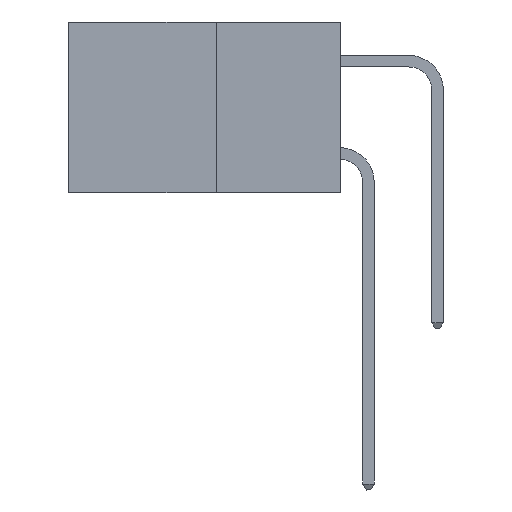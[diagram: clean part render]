
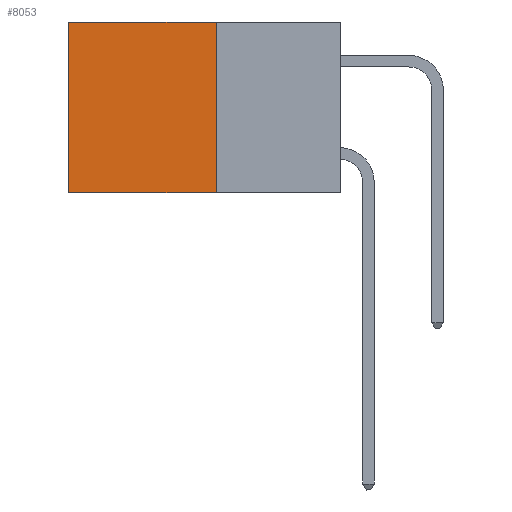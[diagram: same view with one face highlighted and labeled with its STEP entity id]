
A CAD part, left-side view. The second image highlights one B-rep face of the part: STEP entity #8053.
In plain terms, the highlighted planar face has unit normal (-1, 0, 0).
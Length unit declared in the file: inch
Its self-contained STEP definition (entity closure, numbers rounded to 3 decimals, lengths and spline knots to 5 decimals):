
#97 = CARTESIAN_POINT ( 'NONE',  ( 0.277, 0.59, 0. ) ) ;
#170 = EDGE_CURVE ( 'NONE', #8629, #263, #5665, .T. ) ;
#263 = VERTEX_POINT ( 'NONE', #1563 ) ;
#1008 = VECTOR ( 'NONE', #2138, 39.37008 ) ;
#1126 = ORIENTED_EDGE ( 'NONE', *, *, #170, .T. ) ;
#1205 = EDGE_LOOP ( 'NONE', ( #1126, #2444, #7667, #8447 ) ) ;
#1517 = VERTEX_POINT ( 'NONE', #9503 ) ;
#1563 = CARTESIAN_POINT ( 'NONE',  ( 0.277, 0.59, -0.37 ) ) ;
#2138 = DIRECTION ( 'NONE',  ( 0., 0., -1. ) ) ;
#2444 = ORIENTED_EDGE ( 'NONE', *, *, #2833, .F. ) ;
#2833 = EDGE_CURVE ( 'NONE', #4361, #263, #10148, .T. ) ;
#3329 = LINE ( 'NONE', #5433, #7094 ) ;
#4015 = AXIS2_PLACEMENT_3D ( 'NONE', #7251, #4735, #4480 ) ;
#4361 = VERTEX_POINT ( 'NONE', #9596 ) ;
#4480 = DIRECTION ( 'NONE',  ( 0., 0., -1. ) ) ;
#4735 = DIRECTION ( 'NONE',  ( 1., 0., 0. ) ) ;
#5254 = PLANE ( 'NONE',  #4015 ) ;
#5394 = VECTOR ( 'NONE', #8685, 39.37008 ) ;
#5433 = CARTESIAN_POINT ( 'NONE',  ( 0.277, 0.27, -0.37 ) ) ;
#5443 = CARTESIAN_POINT ( 'NONE',  ( 0.277, 0.27, -0.37 ) ) ;
#5665 = LINE ( 'NONE', #7235, #1008 ) ;
#6335 = DIRECTION ( 'NONE',  ( 0., 0., -1. ) ) ;
#7041 = FACE_OUTER_BOUND ( 'NONE', #1205, .T. ) ;
#7094 = VECTOR ( 'NONE', #6335, 39.37008 ) ;
#7235 = CARTESIAN_POINT ( 'NONE',  ( 0.277, 0.59, -0.37 ) ) ;
#7251 = CARTESIAN_POINT ( 'NONE',  ( 0.277, 0.27, -0.37 ) ) ;
#7667 = ORIENTED_EDGE ( 'NONE', *, *, #8996, .F. ) ;
#7945 = VECTOR ( 'NONE', #10150, 39.37008 ) ;
#8053 = ADVANCED_FACE ( 'NONE', ( #7041 ), #5254, .F. ) ;
#8196 = EDGE_CURVE ( 'NONE', #1517, #8629, #9662, .T. ) ;
#8447 = ORIENTED_EDGE ( 'NONE', *, *, #8196, .T. ) ;
#8629 = VERTEX_POINT ( 'NONE', #97 ) ;
#8685 = DIRECTION ( 'NONE',  ( 0., 1., 0. ) ) ;
#8731 = CARTESIAN_POINT ( 'NONE',  ( 0.277, 0.27, 0. ) ) ;
#8996 = EDGE_CURVE ( 'NONE', #1517, #4361, #3329, .T. ) ;
#9503 = CARTESIAN_POINT ( 'NONE',  ( 0.277, 0.27, 0. ) ) ;
#9596 = CARTESIAN_POINT ( 'NONE',  ( 0.277, 0.27, -0.37 ) ) ;
#9662 = LINE ( 'NONE', #8731, #5394 ) ;
#10148 = LINE ( 'NONE', #5443, #7945 ) ;
#10150 = DIRECTION ( 'NONE',  ( 0., 1., 0. ) ) ;
